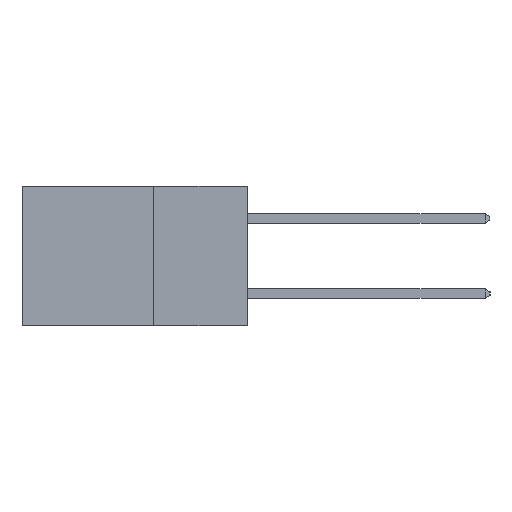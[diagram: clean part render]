
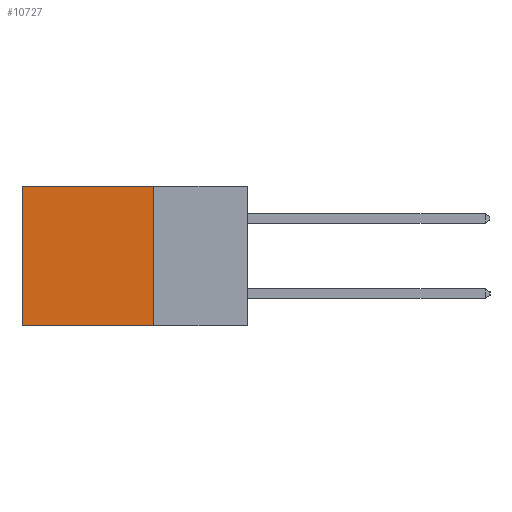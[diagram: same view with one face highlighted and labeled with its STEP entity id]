
A CAD part, left-side view. The second image highlights one B-rep face of the part: STEP entity #10727.
In plain terms, the highlighted planar face has unit normal (-1, 0, 0).
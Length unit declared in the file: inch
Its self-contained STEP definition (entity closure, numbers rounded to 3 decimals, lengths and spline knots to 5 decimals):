
#207 = VERTEX_POINT ( 'NONE', #2433 ) ;
#570 = VECTOR ( 'NONE', #3219, 39.37008 ) ;
#874 = DIRECTION ( 'NONE',  ( 0., 1., 0. ) ) ;
#1065 = DIRECTION ( 'NONE',  ( 0., 0., -1. ) ) ;
#1174 = CARTESIAN_POINT ( 'NONE',  ( 0.2615, 0.6, -0.37 ) ) ;
#1324 = EDGE_CURVE ( 'NONE', #11202, #207, #6885, .T. ) ;
#1918 = CARTESIAN_POINT ( 'NONE',  ( 0.2615, 0.25, 0. ) ) ;
#2433 = CARTESIAN_POINT ( 'NONE',  ( 0.2615, 0.25, -0.37 ) ) ;
#2850 = VERTEX_POINT ( 'NONE', #8198 ) ;
#3023 = DIRECTION ( 'NONE',  ( 0., 0., -1. ) ) ;
#3071 = DIRECTION ( 'NONE',  ( 1., 0., 0. ) ) ;
#3108 = PLANE ( 'NONE',  #5428 ) ;
#3219 = DIRECTION ( 'NONE',  ( 0., 1., 0. ) ) ;
#3378 = CARTESIAN_POINT ( 'NONE',  ( 0.2615, 0.25, -0.37 ) ) ;
#3742 = VECTOR ( 'NONE', #14485, 39.37008 ) ;
#4361 = CARTESIAN_POINT ( 'NONE',  ( 0.2615, 0.25, -0.37 ) ) ;
#4566 = ORIENTED_EDGE ( 'NONE', *, *, #7817, .F. ) ;
#4761 = EDGE_CURVE ( 'NONE', #2850, #7744, #8816, .T. ) ;
#4792 = LINE ( 'NONE', #1918, #10647 ) ;
#5314 = CARTESIAN_POINT ( 'NONE',  ( 0.2615, 0.6, -0.37 ) ) ;
#5428 = AXIS2_PLACEMENT_3D ( 'NONE', #3378, #3071, #3023 ) ;
#6885 = LINE ( 'NONE', #14398, #3742 ) ;
#7744 = VERTEX_POINT ( 'NONE', #5314 ) ;
#7817 = EDGE_CURVE ( 'NONE', #207, #7744, #9992, .T. ) ;
#8198 = CARTESIAN_POINT ( 'NONE',  ( 0.2615, 0.6, 0. ) ) ;
#8545 = ORIENTED_EDGE ( 'NONE', *, *, #10789, .T. ) ;
#8816 = LINE ( 'NONE', #1174, #11165 ) ;
#9142 = ORIENTED_EDGE ( 'NONE', *, *, #4761, .T. ) ;
#9992 = LINE ( 'NONE', #4361, #570 ) ;
#10647 = VECTOR ( 'NONE', #874, 39.37008 ) ;
#10727 = ADVANCED_FACE ( 'NONE', ( #14224 ), #3108, .F. ) ;
#10789 = EDGE_CURVE ( 'NONE', #11202, #2850, #4792, .T. ) ;
#11165 = VECTOR ( 'NONE', #1065, 39.37008 ) ;
#11202 = VERTEX_POINT ( 'NONE', #12179 ) ;
#12179 = CARTESIAN_POINT ( 'NONE',  ( 0.2615, 0.25, 0. ) ) ;
#13755 = EDGE_LOOP ( 'NONE', ( #9142, #4566, #14407, #8545 ) ) ;
#14224 = FACE_OUTER_BOUND ( 'NONE', #13755, .T. ) ;
#14398 = CARTESIAN_POINT ( 'NONE',  ( 0.2615, 0.25, -0.37 ) ) ;
#14407 = ORIENTED_EDGE ( 'NONE', *, *, #1324, .F. ) ;
#14485 = DIRECTION ( 'NONE',  ( 0., 0., -1. ) ) ;
